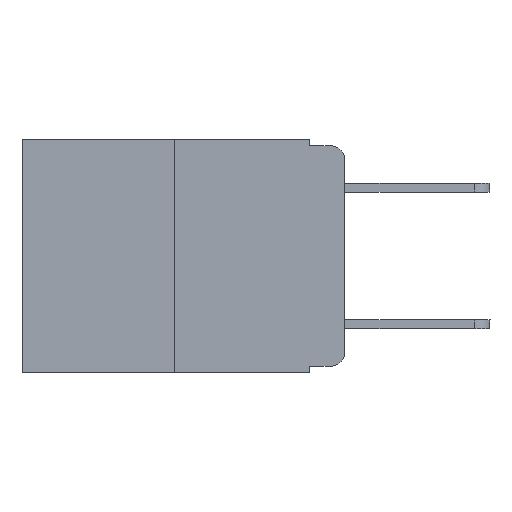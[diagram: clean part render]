
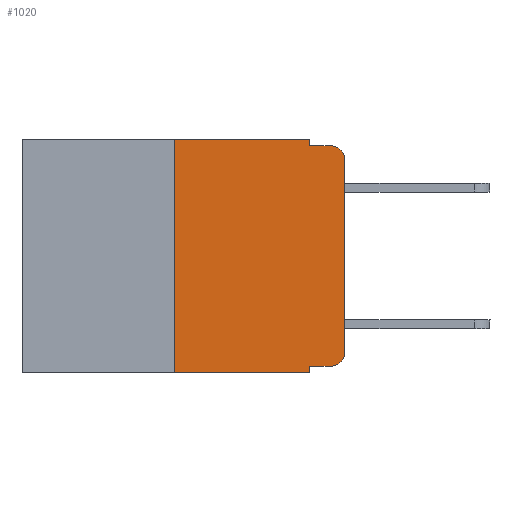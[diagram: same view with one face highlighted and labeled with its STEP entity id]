
A CAD part, left-side view. The second image highlights one B-rep face of the part: STEP entity #1020.
In plain terms, the highlighted planar face has unit normal (-1, 0, 0).
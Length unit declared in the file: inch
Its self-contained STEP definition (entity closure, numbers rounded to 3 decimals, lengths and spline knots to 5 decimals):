
#10 = LINE ( 'NONE', #6640, #9914 ) ;
#353 = CARTESIAN_POINT ( 'NONE',  ( 0., 0., -0.313 ) ) ;
#718 = CARTESIAN_POINT ( 'NONE',  ( 0., 0.25, -0.343 ) ) ;
#831 = VECTOR ( 'NONE', #14280, 39.37008 ) ;
#1020 = ADVANCED_FACE ( 'NONE', ( #10602 ), #13763, .F. ) ;
#1073 = CARTESIAN_POINT ( 'NONE',  ( 0., 0.02, -0.03 ) ) ;
#1078 = LINE ( 'NONE', #5397, #6407 ) ;
#1156 = DIRECTION ( 'NONE',  ( 0., -1., 0. ) ) ;
#1402 = CARTESIAN_POINT ( 'NONE',  ( 0., 0.25, 0. ) ) ;
#1432 = CARTESIAN_POINT ( 'NONE',  ( 0., 0.051, -0.01 ) ) ;
#1475 = ORIENTED_EDGE ( 'NONE', *, *, #10126, .T. ) ;
#2015 = LINE ( 'NONE', #6463, #831 ) ;
#2031 = EDGE_CURVE ( 'NONE', #4165, #2866, #8339, .T. ) ;
#2117 = DIRECTION ( 'NONE',  ( 0., 0., -1. ) ) ;
#2171 = DIRECTION ( 'NONE',  ( 0., 0., -1. ) ) ;
#2175 = CARTESIAN_POINT ( 'NONE',  ( 0., 0., -0.03 ) ) ;
#2229 = DIRECTION ( 'NONE',  ( 0., -1., 0. ) ) ;
#2312 = VECTOR ( 'NONE', #1156, 39.37008 ) ;
#2866 = VERTEX_POINT ( 'NONE', #7034 ) ;
#2940 = VERTEX_POINT ( 'NONE', #353 ) ;
#3174 = LINE ( 'NONE', #13273, #14051 ) ;
#3212 = AXIS2_PLACEMENT_3D ( 'NONE', #13762, #3691, #7195 ) ;
#3511 = ORIENTED_EDGE ( 'NONE', *, *, #2031, .F. ) ;
#3636 = ORIENTED_EDGE ( 'NONE', *, *, #4600, .F. ) ;
#3691 = DIRECTION ( 'NONE',  ( -1., 0., 0. ) ) ;
#3766 = VERTEX_POINT ( 'NONE', #1432 ) ;
#3823 = CARTESIAN_POINT ( 'NONE',  ( 0., 0.473, 0. ) ) ;
#3977 = CARTESIAN_POINT ( 'NONE',  ( 0., 0.051, -0.333 ) ) ;
#4165 = VERTEX_POINT ( 'NONE', #6688 ) ;
#4583 = CIRCLE ( 'NONE', #12701, 0.02 ) ;
#4600 = EDGE_CURVE ( 'NONE', #2866, #3766, #3174, .T. ) ;
#4669 = EDGE_LOOP ( 'NONE', ( #13996, #9410, #5178, #3636, #3511, #13623, #9128, #12391, #1475, #11301 ) ) ;
#4681 = CARTESIAN_POINT ( 'NONE',  ( 0., 0.02, -0.333 ) ) ;
#4687 = AXIS2_PLACEMENT_3D ( 'NONE', #3823, #8146, #5675 ) ;
#5041 = EDGE_CURVE ( 'NONE', #6047, #13379, #4583, .T. ) ;
#5178 = ORIENTED_EDGE ( 'NONE', *, *, #8344, .F. ) ;
#5397 = CARTESIAN_POINT ( 'NONE',  ( 0., 0.051, 0. ) ) ;
#5525 = LINE ( 'NONE', #6614, #6477 ) ;
#5557 = DIRECTION ( 'NONE',  ( 0., -1., 0. ) ) ;
#5675 = DIRECTION ( 'NONE',  ( 0., 0., -1. ) ) ;
#5961 = VECTOR ( 'NONE', #8050, 39.37008 ) ;
#6047 = VERTEX_POINT ( 'NONE', #2175 ) ;
#6103 = EDGE_CURVE ( 'NONE', #10456, #11842, #1078, .T. ) ;
#6119 = LINE ( 'NONE', #11865, #9443 ) ;
#6407 = VECTOR ( 'NONE', #2117, 39.37008 ) ;
#6463 = CARTESIAN_POINT ( 'NONE',  ( 0., 0.051, -0.01 ) ) ;
#6477 = VECTOR ( 'NONE', #2229, 39.37008 ) ;
#6614 = CARTESIAN_POINT ( 'NONE',  ( 0., 0.051, -0.333 ) ) ;
#6640 = CARTESIAN_POINT ( 'NONE',  ( 0., 0.473, -0.343 ) ) ;
#6688 = CARTESIAN_POINT ( 'NONE',  ( 0., 0.25, 0. ) ) ;
#7034 = CARTESIAN_POINT ( 'NONE',  ( 0., 0.051, 0. ) ) ;
#7195 = DIRECTION ( 'NONE',  ( 0., 0., -1. ) ) ;
#8050 = DIRECTION ( 'NONE',  ( 0., 0., 1. ) ) ;
#8146 = DIRECTION ( 'NONE',  ( 1., 0., 0. ) ) ;
#8339 = LINE ( 'NONE', #9339, #2312 ) ;
#8344 = EDGE_CURVE ( 'NONE', #3766, #13379, #2015, .T. ) ;
#8385 = DIRECTION ( 'NONE',  ( 0., 0., 1. ) ) ;
#8706 = EDGE_CURVE ( 'NONE', #12621, #11842, #10, .T. ) ;
#9128 = ORIENTED_EDGE ( 'NONE', *, *, #8706, .T. ) ;
#9339 = CARTESIAN_POINT ( 'NONE',  ( 0., 0.473, 0. ) ) ;
#9410 = ORIENTED_EDGE ( 'NONE', *, *, #5041, .T. ) ;
#9443 = VECTOR ( 'NONE', #8385, 39.37008 ) ;
#9560 = CARTESIAN_POINT ( 'NONE',  ( 0., 0.02, -0.01 ) ) ;
#9914 = VECTOR ( 'NONE', #5557, 39.37008 ) ;
#10126 = EDGE_CURVE ( 'NONE', #10456, #13660, #5525, .T. ) ;
#10237 = EDGE_CURVE ( 'NONE', #13660, #2940, #13865, .T. ) ;
#10242 = LINE ( 'NONE', #1402, #5961 ) ;
#10456 = VERTEX_POINT ( 'NONE', #3977 ) ;
#10602 = FACE_OUTER_BOUND ( 'NONE', #4669, .T. ) ;
#10971 = DIRECTION ( 'NONE',  ( 0., 0., -1. ) ) ;
#11301 = ORIENTED_EDGE ( 'NONE', *, *, #10237, .T. ) ;
#11842 = VERTEX_POINT ( 'NONE', #13487 ) ;
#11865 = CARTESIAN_POINT ( 'NONE',  ( 0., 0., 0. ) ) ;
#11997 = EDGE_CURVE ( 'NONE', #12621, #4165, #10242, .T. ) ;
#12391 = ORIENTED_EDGE ( 'NONE', *, *, #6103, .F. ) ;
#12594 = EDGE_CURVE ( 'NONE', #2940, #6047, #6119, .T. ) ;
#12621 = VERTEX_POINT ( 'NONE', #718 ) ;
#12701 = AXIS2_PLACEMENT_3D ( 'NONE', #1073, #14307, #2171 ) ;
#13273 = CARTESIAN_POINT ( 'NONE',  ( 0., 0.051, 0. ) ) ;
#13379 = VERTEX_POINT ( 'NONE', #9560 ) ;
#13487 = CARTESIAN_POINT ( 'NONE',  ( 0., 0.051, -0.343 ) ) ;
#13623 = ORIENTED_EDGE ( 'NONE', *, *, #11997, .F. ) ;
#13660 = VERTEX_POINT ( 'NONE', #4681 ) ;
#13762 = CARTESIAN_POINT ( 'NONE',  ( 0., 0.02, -0.313 ) ) ;
#13763 = PLANE ( 'NONE',  #4687 ) ;
#13865 = CIRCLE ( 'NONE', #3212, 0.02 ) ;
#13996 = ORIENTED_EDGE ( 'NONE', *, *, #12594, .T. ) ;
#14051 = VECTOR ( 'NONE', #10971, 39.37008 ) ;
#14280 = DIRECTION ( 'NONE',  ( 0., -1., 0. ) ) ;
#14307 = DIRECTION ( 'NONE',  ( -1., 0., 0. ) ) ;
